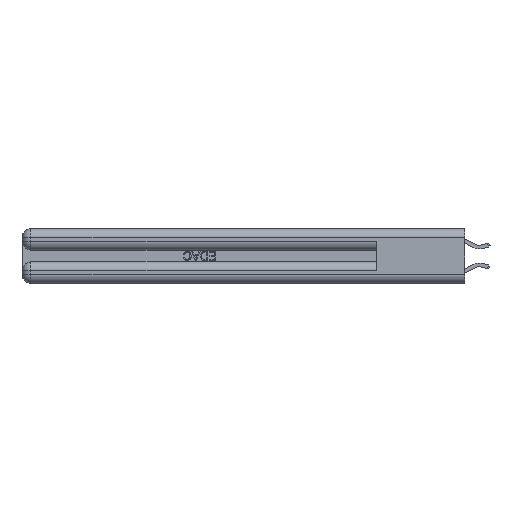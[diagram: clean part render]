
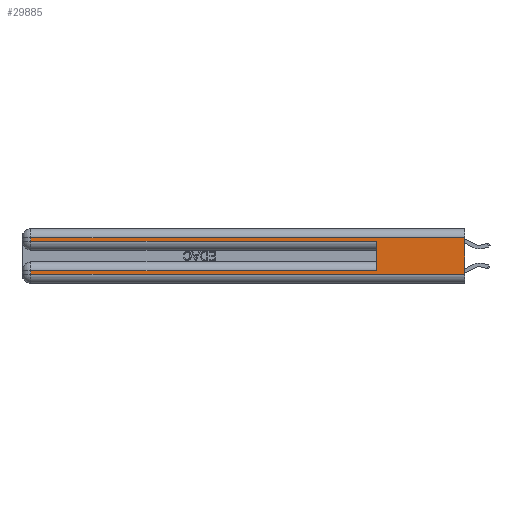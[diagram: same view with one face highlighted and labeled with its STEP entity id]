
A CAD part, left-side view. The second image highlights one B-rep face of the part: STEP entity #29885.
In plain terms, the highlighted planar face has unit normal (-1, 0, 0).
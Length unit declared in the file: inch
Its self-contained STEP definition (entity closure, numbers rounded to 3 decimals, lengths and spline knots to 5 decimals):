
#97 = EDGE_LOOP ( 'NONE', ( #30605, #31102, #21006, #4831, #13462, #14763, #13199, #23133 ) ) ;
#586 = EDGE_CURVE ( 'NONE', #9076, #5405, #5906, .T. ) ;
#1230 = DIRECTION ( 'NONE',  ( 0., 0., -1. ) ) ;
#2006 = VECTOR ( 'NONE', #12057, 39.37008 ) ;
#2458 = PLANE ( 'NONE',  #21406 ) ;
#2603 = CARTESIAN_POINT ( 'NONE',  ( 0., 0., 0.31 ) ) ;
#2773 = LINE ( 'NONE', #4731, #2006 ) ;
#3321 = LINE ( 'NONE', #13129, #17159 ) ;
#3837 = FACE_OUTER_BOUND ( 'NONE', #97, .T. ) ;
#4731 = CARTESIAN_POINT ( 'NONE',  ( 0., 0.6, 0.145 ) ) ;
#4831 = ORIENTED_EDGE ( 'NONE', *, *, #6361, .T. ) ;
#5405 = VERTEX_POINT ( 'NONE', #21755 ) ;
#5729 = VECTOR ( 'NONE', #21964, 39.37008 ) ;
#5820 = VERTEX_POINT ( 'NONE', #22269 ) ;
#5906 = LINE ( 'NONE', #25198, #14007 ) ;
#6361 = EDGE_CURVE ( 'NONE', #5820, #18485, #10197, .T. ) ;
#6401 = LINE ( 'NONE', #7167, #18723 ) ;
#6520 = CARTESIAN_POINT ( 'NONE',  ( 0., 0.6, 0.285 ) ) ;
#7167 = CARTESIAN_POINT ( 'NONE',  ( 0., 0., 0.37 ) ) ;
#8321 = VERTEX_POINT ( 'NONE', #14958 ) ;
#8370 = EDGE_CURVE ( 'NONE', #9076, #18485, #2773, .T. ) ;
#9076 = VERTEX_POINT ( 'NONE', #18724 ) ;
#9204 = LINE ( 'NONE', #24766, #5729 ) ;
#9841 = EDGE_CURVE ( 'NONE', #23208, #8321, #25792, .T. ) ;
#10197 = LINE ( 'NONE', #16674, #19422 ) ;
#12057 = DIRECTION ( 'NONE',  ( 0., 0., 1. ) ) ;
#12290 = EDGE_CURVE ( 'NONE', #5405, #21124, #22920, .T. ) ;
#12452 = DIRECTION ( 'NONE',  ( 0., 0., -1. ) ) ;
#13129 = CARTESIAN_POINT ( 'NONE',  ( 0., 2.94, 0.37 ) ) ;
#13199 = ORIENTED_EDGE ( 'NONE', *, *, #12290, .T. ) ;
#13462 = ORIENTED_EDGE ( 'NONE', *, *, #8370, .F. ) ;
#14007 = VECTOR ( 'NONE', #18141, 39.37008 ) ;
#14763 = ORIENTED_EDGE ( 'NONE', *, *, #586, .T. ) ;
#14958 = CARTESIAN_POINT ( 'NONE',  ( 0., 2.94, 0.31 ) ) ;
#15779 = CARTESIAN_POINT ( 'NONE',  ( 0., 2.94, 0.06 ) ) ;
#16674 = CARTESIAN_POINT ( 'NONE',  ( 0., 0., 0.285 ) ) ;
#16740 = DIRECTION ( 'NONE',  ( 0., 1., 0. ) ) ;
#17159 = VECTOR ( 'NONE', #25242, 39.37008 ) ;
#17258 = DIRECTION ( 'NONE',  ( 0., 0., -1. ) ) ;
#18110 = CARTESIAN_POINT ( 'NONE',  ( 0., 0., 0.06 ) ) ;
#18141 = DIRECTION ( 'NONE',  ( 0., 1., 0. ) ) ;
#18485 = VERTEX_POINT ( 'NONE', #6520 ) ;
#18723 = VECTOR ( 'NONE', #17258, 39.37008 ) ;
#18724 = CARTESIAN_POINT ( 'NONE',  ( 0., 0.6, 0.085 ) ) ;
#18810 = EDGE_CURVE ( 'NONE', #21124, #23992, #9204, .T. ) ;
#19422 = VECTOR ( 'NONE', #24282, 39.37008 ) ;
#20553 = CARTESIAN_POINT ( 'NONE',  ( 0., 2.94, 0.37 ) ) ;
#21006 = ORIENTED_EDGE ( 'NONE', *, *, #21590, .T. ) ;
#21124 = VERTEX_POINT ( 'NONE', #15779 ) ;
#21406 = AXIS2_PLACEMENT_3D ( 'NONE', #22081, #29202, #12452 ) ;
#21590 = EDGE_CURVE ( 'NONE', #8321, #5820, #3321, .T. ) ;
#21755 = CARTESIAN_POINT ( 'NONE',  ( 0., 2.94, 0.085 ) ) ;
#21923 = VECTOR ( 'NONE', #16740, 39.37008 ) ;
#21964 = DIRECTION ( 'NONE',  ( 0., -1., 0. ) ) ;
#22081 = CARTESIAN_POINT ( 'NONE',  ( 0., 0., 0.37 ) ) ;
#22269 = CARTESIAN_POINT ( 'NONE',  ( 0., 2.94, 0.285 ) ) ;
#22519 = EDGE_CURVE ( 'NONE', #23208, #23992, #6401, .T. ) ;
#22920 = LINE ( 'NONE', #20553, #24460 ) ;
#23133 = ORIENTED_EDGE ( 'NONE', *, *, #18810, .T. ) ;
#23208 = VERTEX_POINT ( 'NONE', #2603 ) ;
#23992 = VERTEX_POINT ( 'NONE', #18110 ) ;
#24282 = DIRECTION ( 'NONE',  ( 0., -1., 0. ) ) ;
#24460 = VECTOR ( 'NONE', #1230, 39.37008 ) ;
#24766 = CARTESIAN_POINT ( 'NONE',  ( 0., 0., 0.06 ) ) ;
#25198 = CARTESIAN_POINT ( 'NONE',  ( 0., 0., 0.085 ) ) ;
#25242 = DIRECTION ( 'NONE',  ( 0., 0., -1. ) ) ;
#25792 = LINE ( 'NONE', #29299, #21923 ) ;
#29202 = DIRECTION ( 'NONE',  ( 1., 0., 0. ) ) ;
#29299 = CARTESIAN_POINT ( 'NONE',  ( 0., 0., 0.31 ) ) ;
#29885 = ADVANCED_FACE ( 'NONE', ( #3837 ), #2458, .F. ) ;
#30605 = ORIENTED_EDGE ( 'NONE', *, *, #22519, .F. ) ;
#31102 = ORIENTED_EDGE ( 'NONE', *, *, #9841, .T. ) ;
